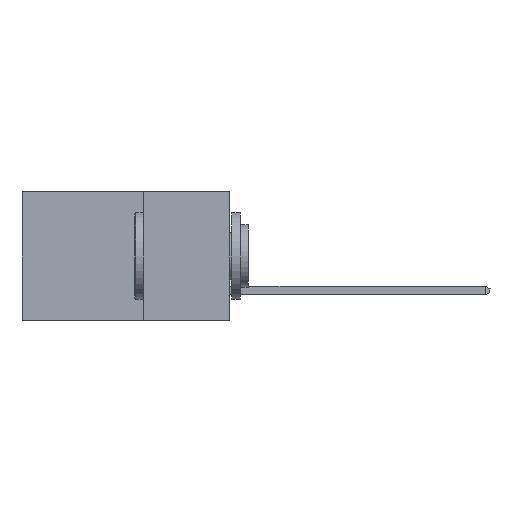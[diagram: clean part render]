
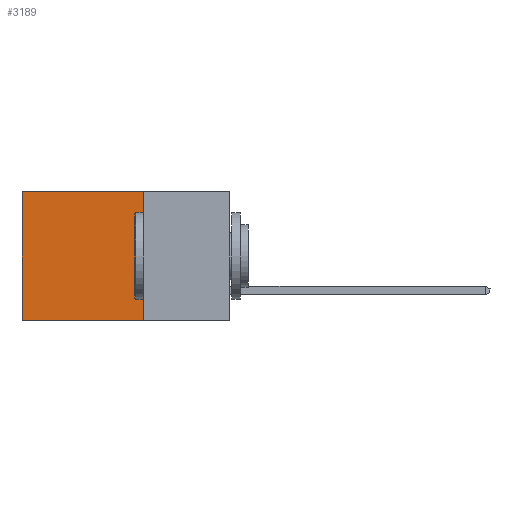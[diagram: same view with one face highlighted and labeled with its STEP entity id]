
A CAD part, left-side view. The second image highlights one B-rep face of the part: STEP entity #3189.
In plain terms, the highlighted planar face has unit normal (-1, 0, 0).
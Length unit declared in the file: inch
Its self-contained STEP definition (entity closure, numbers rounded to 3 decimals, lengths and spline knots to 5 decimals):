
#184 = VERTEX_POINT ( 'NONE', #9016 ) ;
#461 = EDGE_LOOP ( 'NONE', ( #8295, #943, #10038, #11579 ) ) ;
#943 = ORIENTED_EDGE ( 'NONE', *, *, #3771, .F. ) ;
#1876 = AXIS2_PLACEMENT_3D ( 'NONE', #8238, #7319, #6399 ) ;
#2385 = CARTESIAN_POINT ( 'NONE',  ( 0.2615, 0.25, -0.37 ) ) ;
#3063 = VECTOR ( 'NONE', #7931, 39.37008 ) ;
#3073 = VECTOR ( 'NONE', #11486, 39.37008 ) ;
#3189 = ADVANCED_FACE ( 'NONE', ( #3631 ), #6578, .F. ) ;
#3264 = CARTESIAN_POINT ( 'NONE',  ( 0.2615, 0.6, -0.37 ) ) ;
#3305 = DIRECTION ( 'NONE',  ( 0., 0., -1. ) ) ;
#3574 = VECTOR ( 'NONE', #3305, 39.37008 ) ;
#3631 = FACE_OUTER_BOUND ( 'NONE', #461, .T. ) ;
#3771 = EDGE_CURVE ( 'NONE', #8554, #9596, #4447, .T. ) ;
#3965 = LINE ( 'NONE', #7721, #3073 ) ;
#3999 = LINE ( 'NONE', #2385, #3063 ) ;
#4447 = LINE ( 'NONE', #8928, #9021 ) ;
#5244 = EDGE_CURVE ( 'NONE', #7532, #9596, #8828, .T. ) ;
#5540 = EDGE_CURVE ( 'NONE', #184, #7532, #3965, .T. ) ;
#6399 = DIRECTION ( 'NONE',  ( 0., 0., -1. ) ) ;
#6578 = PLANE ( 'NONE',  #1876 ) ;
#7319 = DIRECTION ( 'NONE',  ( 1., 0., 0. ) ) ;
#7532 = VERTEX_POINT ( 'NONE', #11969 ) ;
#7721 = CARTESIAN_POINT ( 'NONE',  ( 0.2615, 0.25, 0. ) ) ;
#7931 = DIRECTION ( 'NONE',  ( 0., 0., -1. ) ) ;
#8238 = CARTESIAN_POINT ( 'NONE',  ( 0.2615, 0.25, -0.37 ) ) ;
#8295 = ORIENTED_EDGE ( 'NONE', *, *, #5244, .T. ) ;
#8554 = VERTEX_POINT ( 'NONE', #9509 ) ;
#8828 = LINE ( 'NONE', #11686, #3574 ) ;
#8928 = CARTESIAN_POINT ( 'NONE',  ( 0.2615, 0.25, -0.37 ) ) ;
#9016 = CARTESIAN_POINT ( 'NONE',  ( 0.2615, 0.25, 0. ) ) ;
#9021 = VECTOR ( 'NONE', #11905, 39.37008 ) ;
#9509 = CARTESIAN_POINT ( 'NONE',  ( 0.2615, 0.25, -0.37 ) ) ;
#9593 = EDGE_CURVE ( 'NONE', #184, #8554, #3999, .T. ) ;
#9596 = VERTEX_POINT ( 'NONE', #3264 ) ;
#10038 = ORIENTED_EDGE ( 'NONE', *, *, #9593, .F. ) ;
#11486 = DIRECTION ( 'NONE',  ( 0., 1., 0. ) ) ;
#11579 = ORIENTED_EDGE ( 'NONE', *, *, #5540, .T. ) ;
#11686 = CARTESIAN_POINT ( 'NONE',  ( 0.2615, 0.6, -0.37 ) ) ;
#11905 = DIRECTION ( 'NONE',  ( 0., 1., 0. ) ) ;
#11969 = CARTESIAN_POINT ( 'NONE',  ( 0.2615, 0.6, 0. ) ) ;
